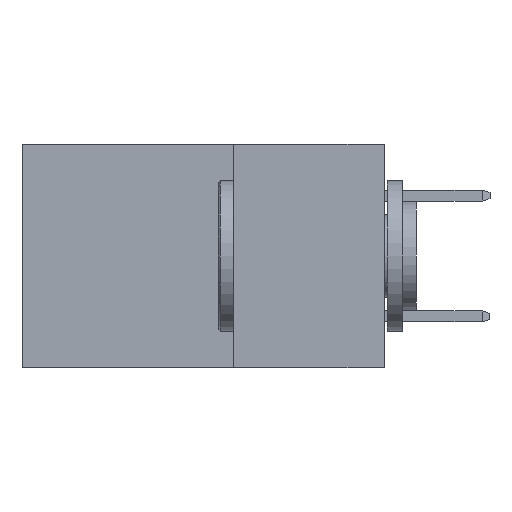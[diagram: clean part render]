
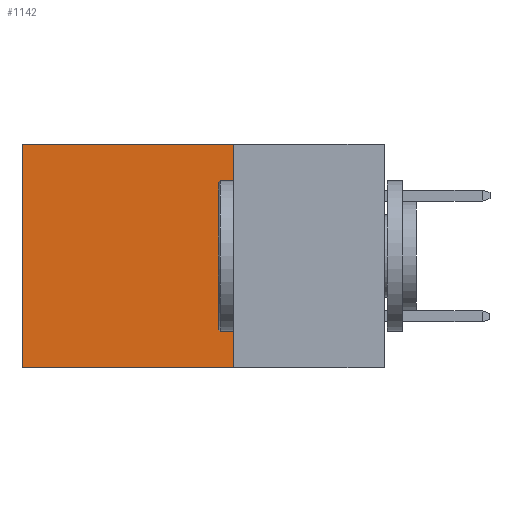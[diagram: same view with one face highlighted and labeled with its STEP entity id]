
A CAD part, left-side view. The second image highlights one B-rep face of the part: STEP entity #1142.
In plain terms, the highlighted planar face has unit normal (-1, 0, 0).
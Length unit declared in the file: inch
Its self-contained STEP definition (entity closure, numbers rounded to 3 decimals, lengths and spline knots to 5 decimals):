
#201 = LINE ( 'NONE', #19251, #27536 ) ;
#279 = CARTESIAN_POINT ( 'NONE',  ( 0.298, 0.25, 0. ) ) ;
#986 = CARTESIAN_POINT ( 'NONE',  ( 0.298, 0.25, 0. ) ) ;
#1142 = ADVANCED_FACE ( 'NONE', ( #18483 ), #18528, .F. ) ;
#2613 = AXIS2_PLACEMENT_3D ( 'NONE', #279, #28987, #15190 ) ;
#2941 = CARTESIAN_POINT ( 'NONE',  ( 0.298, 0.6, -0.37 ) ) ;
#3349 = VERTEX_POINT ( 'NONE', #13521 ) ;
#3736 = ORIENTED_EDGE ( 'NONE', *, *, #18364, .T. ) ;
#4752 = ORIENTED_EDGE ( 'NONE', *, *, #9249, .T. ) ;
#5482 = CARTESIAN_POINT ( 'NONE',  ( 0.298, 0.25, -0.37 ) ) ;
#5559 = VERTEX_POINT ( 'NONE', #23286 ) ;
#6128 = VECTOR ( 'NONE', #7069, 39.37008 ) ;
#7069 = DIRECTION ( 'NONE',  ( 0., 0., -1. ) ) ;
#7236 = EDGE_CURVE ( 'NONE', #3349, #13636, #28000, .T. ) ;
#7524 = LINE ( 'NONE', #14429, #13677 ) ;
#7930 = DIRECTION ( 'NONE',  ( 0., 1., 0. ) ) ;
#9249 = EDGE_CURVE ( 'NONE', #21517, #5559, #7524, .T. ) ;
#9445 = VECTOR ( 'NONE', #7930, 39.37008 ) ;
#10394 = EDGE_CURVE ( 'NONE', #21517, #3349, #25467, .T. ) ;
#12768 = EDGE_LOOP ( 'NONE', ( #3736, #13391, #18351, #4752 ) ) ;
#13391 = ORIENTED_EDGE ( 'NONE', *, *, #7236, .F. ) ;
#13521 = CARTESIAN_POINT ( 'NONE',  ( 0.298, 0.25, -0.37 ) ) ;
#13636 = VERTEX_POINT ( 'NONE', #2941 ) ;
#13677 = VECTOR ( 'NONE', #16783, 39.37008 ) ;
#14429 = CARTESIAN_POINT ( 'NONE',  ( 0.298, 0.25, 0. ) ) ;
#14517 = DIRECTION ( 'NONE',  ( 0., 0., -1. ) ) ;
#15190 = DIRECTION ( 'NONE',  ( 0., 0., -1. ) ) ;
#16783 = DIRECTION ( 'NONE',  ( 0., 1., 0. ) ) ;
#18351 = ORIENTED_EDGE ( 'NONE', *, *, #10394, .F. ) ;
#18364 = EDGE_CURVE ( 'NONE', #5559, #13636, #201, .T. ) ;
#18483 = FACE_OUTER_BOUND ( 'NONE', #12768, .T. ) ;
#18528 = PLANE ( 'NONE',  #2613 ) ;
#18696 = CARTESIAN_POINT ( 'NONE',  ( 0.298, 0.25, 0. ) ) ;
#19251 = CARTESIAN_POINT ( 'NONE',  ( 0.298, 0.6, 0. ) ) ;
#21517 = VERTEX_POINT ( 'NONE', #986 ) ;
#23286 = CARTESIAN_POINT ( 'NONE',  ( 0.298, 0.6, 0. ) ) ;
#25467 = LINE ( 'NONE', #18696, #6128 ) ;
#27536 = VECTOR ( 'NONE', #14517, 39.37008 ) ;
#28000 = LINE ( 'NONE', #5482, #9445 ) ;
#28987 = DIRECTION ( 'NONE',  ( 1., 0., 0. ) ) ;
